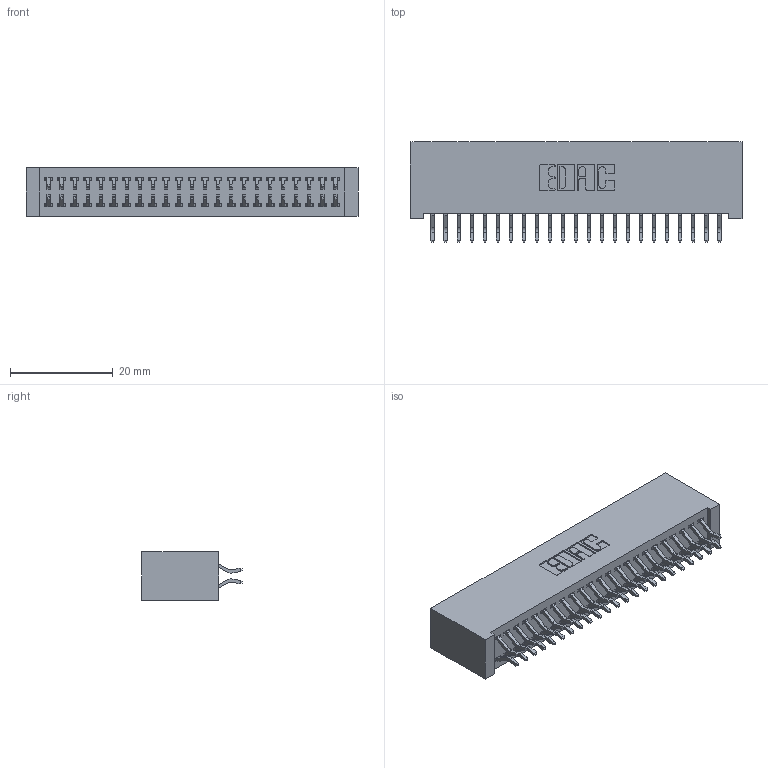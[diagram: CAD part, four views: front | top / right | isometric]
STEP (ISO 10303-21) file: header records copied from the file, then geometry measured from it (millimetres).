
FILE_DESCRIPTION (( 'STEP AP203' ), '1' );
FILE_NAME ('392-046-556-201.STEP', '2018-08-16T19:58:13', ( '' ), ( '' ), 'SwSTEP 2.0', 'SolidWorks 2016', '' );
FILE_SCHEMA (( 'CONFIG_CONTROL_DESIGN' ));
Length unit declared in the file: inch
Products named in the file (3): 342 Part_Lugless; 345-292-001_556 Tail; 392-046-556-201
Assembly tree (47 placements, depth 2):
  392-046-556-201
    342 Part_Lugless
    345-292-001_556 Tail  x46
Bounding box: 64.67 x 19.58 x 9.4 mm (x, y, z)
Volume: 6158.9 mm3; surface area: 9958.5 mm2
Topology: 47 solids, 47 shells, 2770 faces, 8233 edges, 5426 vertices
Faces by surface type: plane 1902, cylinder 868
Entity records: 17065 total; most frequent: CARTESIAN_POINT 2862, ORIENTED_EDGE 2786, DIRECTION 2461, EDGE_CURVE 1393, LINE 1265, VECTOR 1265, VERTEX_POINT 926, AXIS2_PLACEMENT_3D 598
